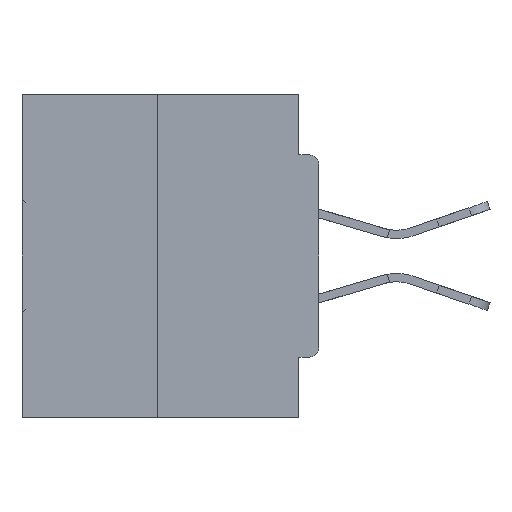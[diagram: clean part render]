
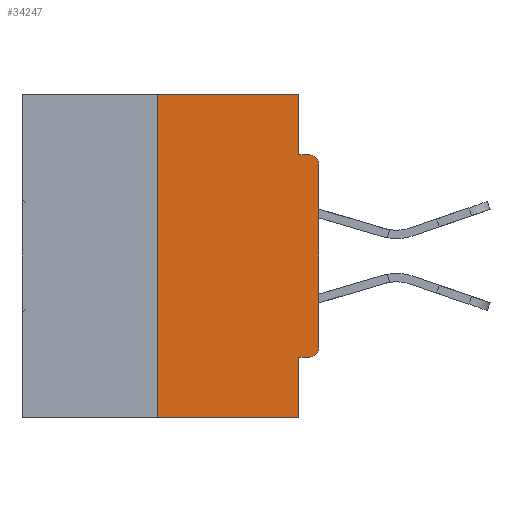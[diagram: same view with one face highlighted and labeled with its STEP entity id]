
A CAD part, left-side view. The second image highlights one B-rep face of the part: STEP entity #34247.
In plain terms, the highlighted planar face has unit normal (-1, 0, 0).
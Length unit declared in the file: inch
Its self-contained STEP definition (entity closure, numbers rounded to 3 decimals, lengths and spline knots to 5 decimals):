
#563 = VERTEX_POINT ( 'NONE', #19584 ) ;
#2597 = DIRECTION ( 'NONE',  ( 0., 0., -1. ) ) ;
#2840 = EDGE_CURVE ( 'NONE', #39892, #40704, #41205, .T. ) ;
#3053 = ORIENTED_EDGE ( 'NONE', *, *, #18698, .T. ) ;
#3080 = DIRECTION ( 'NONE',  ( 0., 0., -1. ) ) ;
#3175 = EDGE_LOOP ( 'NONE', ( #19806, #10556, #3053, #21298, #25476, #42741, #13493, #42923, #40142, #40828 ) ) ;
#3578 = VECTOR ( 'NONE', #32465, 39.37008 ) ;
#3992 = DIRECTION ( 'NONE',  ( 0., 0., -1. ) ) ;
#6206 = CARTESIAN_POINT ( 'NONE',  ( 0., 0.031, 0. ) ) ;
#7763 = CARTESIAN_POINT ( 'NONE',  ( 0., 0.015, -0.4065 ) ) ;
#8336 = VECTOR ( 'NONE', #31350, 39.37008 ) ;
#10556 = ORIENTED_EDGE ( 'NONE', *, *, #15172, .F. ) ;
#10974 = DIRECTION ( 'NONE',  ( 0., -1., 0. ) ) ;
#11310 = VERTEX_POINT ( 'NONE', #11416 ) ;
#11416 = CARTESIAN_POINT ( 'NONE',  ( 0., 0.031, -0.5 ) ) ;
#13007 = DIRECTION ( 'NONE',  ( -1., 0., 0. ) ) ;
#13493 = ORIENTED_EDGE ( 'NONE', *, *, #2840, .T. ) ;
#13544 = VERTEX_POINT ( 'NONE', #25806 ) ;
#13700 = PLANE ( 'NONE',  #34599 ) ;
#13752 = CARTESIAN_POINT ( 'NONE',  ( 0., 0., -0.4065 ) ) ;
#13930 = CARTESIAN_POINT ( 'NONE',  ( 0., 0.25, 0. ) ) ;
#14174 = CARTESIAN_POINT ( 'NONE',  ( 0., 0.031, 0. ) ) ;
#14233 = CIRCLE ( 'NONE', #22197, 0.015 ) ;
#14370 = DIRECTION ( 'NONE',  ( 0., 0., 1. ) ) ;
#14587 = VERTEX_POINT ( 'NONE', #14174 ) ;
#15172 = EDGE_CURVE ( 'NONE', #563, #13544, #34459, .T. ) ;
#16576 = LINE ( 'NONE', #6206, #39350 ) ;
#17511 = CARTESIAN_POINT ( 'NONE',  ( 0., 0., -0.0935 ) ) ;
#18698 = EDGE_CURVE ( 'NONE', #563, #11310, #26713, .T. ) ;
#19584 = CARTESIAN_POINT ( 'NONE',  ( 0., 0.25, -0.5 ) ) ;
#19630 = EDGE_CURVE ( 'NONE', #14587, #27945, #16576, .T. ) ;
#19806 = ORIENTED_EDGE ( 'NONE', *, *, #33991, .F. ) ;
#20196 = DIRECTION ( 'NONE',  ( 0., 0., 1. ) ) ;
#20434 = CARTESIAN_POINT ( 'NONE',  ( 0., 0.015, -0.3915 ) ) ;
#20458 = FACE_OUTER_BOUND ( 'NONE', #3175, .T. ) ;
#20618 = CIRCLE ( 'NONE', #43710, 0.015 ) ;
#21276 = EDGE_CURVE ( 'NONE', #27945, #27528, #34666, .T. ) ;
#21287 = CARTESIAN_POINT ( 'NONE',  ( 0., 0.015, -0.1085 ) ) ;
#21298 = ORIENTED_EDGE ( 'NONE', *, *, #32387, .F. ) ;
#21397 = VECTOR ( 'NONE', #20196, 39.37008 ) ;
#21519 = DIRECTION ( 'NONE',  ( 0., 0., -1. ) ) ;
#21846 = LINE ( 'NONE', #32234, #3578 ) ;
#21999 = DIRECTION ( 'NONE',  ( 0., 0., -1. ) ) ;
#22197 = AXIS2_PLACEMENT_3D ( 'NONE', #20434, #13007, #3080 ) ;
#22663 = VECTOR ( 'NONE', #14370, 39.37008 ) ;
#23355 = EDGE_CURVE ( 'NONE', #35937, #39892, #14233, .T. ) ;
#23775 = DIRECTION ( 'NONE',  ( 0., -1., 0. ) ) ;
#24333 = VECTOR ( 'NONE', #21999, 39.37008 ) ;
#24717 = LINE ( 'NONE', #38736, #24333 ) ;
#25476 = ORIENTED_EDGE ( 'NONE', *, *, #38083, .F. ) ;
#25806 = CARTESIAN_POINT ( 'NONE',  ( 0., 0.25, 0. ) ) ;
#26016 = CARTESIAN_POINT ( 'NONE',  ( 0., 0., -0.3915 ) ) ;
#26713 = LINE ( 'NONE', #44327, #31441 ) ;
#26734 = VERTEX_POINT ( 'NONE', #44535 ) ;
#27528 = VERTEX_POINT ( 'NONE', #28770 ) ;
#27945 = VERTEX_POINT ( 'NONE', #40204 ) ;
#28770 = CARTESIAN_POINT ( 'NONE',  ( 0., 0.015, -0.0935 ) ) ;
#31350 = DIRECTION ( 'NONE',  ( 0., 1., 0. ) ) ;
#31441 = VECTOR ( 'NONE', #23775, 39.37008 ) ;
#32234 = CARTESIAN_POINT ( 'NONE',  ( 0., 0.46, 0. ) ) ;
#32387 = EDGE_CURVE ( 'NONE', #26734, #11310, #24717, .T. ) ;
#32465 = DIRECTION ( 'NONE',  ( 0., -1., 0. ) ) ;
#33991 = EDGE_CURVE ( 'NONE', #13544, #14587, #21846, .T. ) ;
#34247 = ADVANCED_FACE ( 'NONE', ( #20458 ), #13700, .F. ) ;
#34459 = LINE ( 'NONE', #13930, #22663 ) ;
#34599 = AXIS2_PLACEMENT_3D ( 'NONE', #41243, #40555, #3992 ) ;
#34666 = LINE ( 'NONE', #17511, #43050 ) ;
#34862 = CARTESIAN_POINT ( 'NONE',  ( 0., 0., 0. ) ) ;
#35937 = VERTEX_POINT ( 'NONE', #7763 ) ;
#38083 = EDGE_CURVE ( 'NONE', #35937, #26734, #38573, .T. ) ;
#38573 = LINE ( 'NONE', #13752, #8336 ) ;
#38736 = CARTESIAN_POINT ( 'NONE',  ( 0., 0.031, -0.5 ) ) ;
#39129 = EDGE_CURVE ( 'NONE', #40704, #27528, #20618, .T. ) ;
#39350 = VECTOR ( 'NONE', #2597, 39.37008 ) ;
#39706 = CARTESIAN_POINT ( 'NONE',  ( 0., 0., -0.1085 ) ) ;
#39892 = VERTEX_POINT ( 'NONE', #26016 ) ;
#40142 = ORIENTED_EDGE ( 'NONE', *, *, #21276, .F. ) ;
#40204 = CARTESIAN_POINT ( 'NONE',  ( 0., 0.031, -0.0935 ) ) ;
#40555 = DIRECTION ( 'NONE',  ( 1., 0., 0. ) ) ;
#40704 = VERTEX_POINT ( 'NONE', #39706 ) ;
#40828 = ORIENTED_EDGE ( 'NONE', *, *, #19630, .F. ) ;
#41205 = LINE ( 'NONE', #34862, #21397 ) ;
#41243 = CARTESIAN_POINT ( 'NONE',  ( 0., 0.46, 0. ) ) ;
#42741 = ORIENTED_EDGE ( 'NONE', *, *, #23355, .T. ) ;
#42923 = ORIENTED_EDGE ( 'NONE', *, *, #39129, .T. ) ;
#42956 = DIRECTION ( 'NONE',  ( -1., 0., 0. ) ) ;
#43050 = VECTOR ( 'NONE', #10974, 39.37008 ) ;
#43710 = AXIS2_PLACEMENT_3D ( 'NONE', #21287, #42956, #21519 ) ;
#44327 = CARTESIAN_POINT ( 'NONE',  ( 0., 0.46, -0.5 ) ) ;
#44535 = CARTESIAN_POINT ( 'NONE',  ( 0., 0.031, -0.4065 ) ) ;
